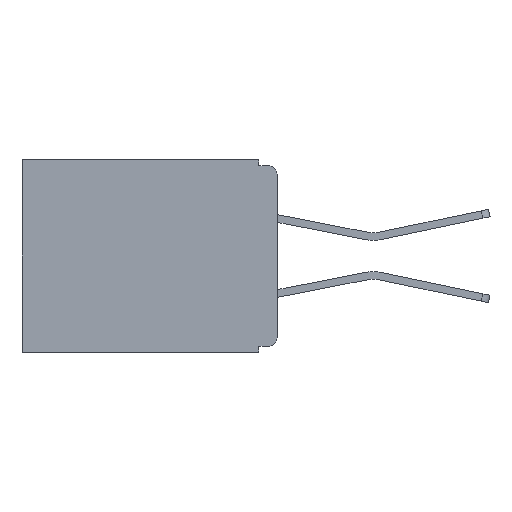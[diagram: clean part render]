
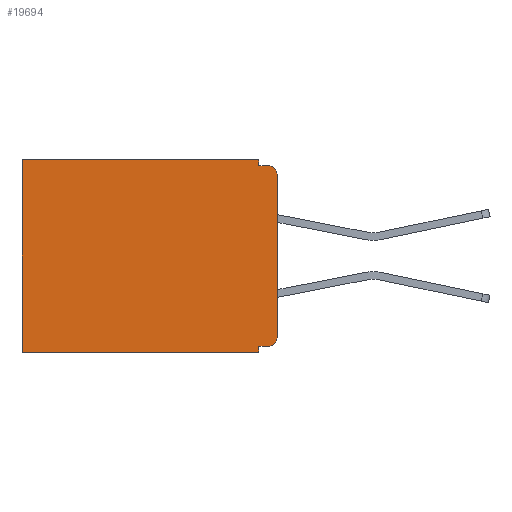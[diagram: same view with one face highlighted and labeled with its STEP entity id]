
A CAD part, left-side view. The second image highlights one B-rep face of the part: STEP entity #19694.
In plain terms, the highlighted planar face has unit normal (-1, 0, 0).
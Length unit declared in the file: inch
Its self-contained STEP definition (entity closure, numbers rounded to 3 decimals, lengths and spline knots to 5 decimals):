
#297 = CARTESIAN_POINT ( 'NONE',  ( 0.3, 0., -0.305 ) ) ;
#701 = LINE ( 'NONE', #4258, #16266 ) ;
#1469 = CARTESIAN_POINT ( 'NONE',  ( 0.3, 0.015, -0.025 ) ) ;
#2181 = DIRECTION ( 'NONE',  ( 0., -1., 0. ) ) ;
#2415 = VECTOR ( 'NONE', #14449, 39.37008 ) ;
#2641 = AXIS2_PLACEMENT_3D ( 'NONE', #9192, #23034, #11213 ) ;
#2864 = EDGE_CURVE ( 'NONE', #6134, #24382, #22647, .T. ) ;
#3348 = ORIENTED_EDGE ( 'NONE', *, *, #19267, .F. ) ;
#3487 = ORIENTED_EDGE ( 'NONE', *, *, #22700, .F. ) ;
#3613 = DIRECTION ( 'NONE',  ( 0., 0., -1. ) ) ;
#3929 = CARTESIAN_POINT ( 'NONE',  ( 0.3, 0., -0.33 ) ) ;
#4196 = ORIENTED_EDGE ( 'NONE', *, *, #20376, .T. ) ;
#4258 = CARTESIAN_POINT ( 'NONE',  ( 0.3, 0.031, -0.33 ) ) ;
#4679 = ORIENTED_EDGE ( 'NONE', *, *, #13429, .F. ) ;
#4730 = CARTESIAN_POINT ( 'NONE',  ( 0.3, 0.031, 0. ) ) ;
#5563 = ORIENTED_EDGE ( 'NONE', *, *, #15061, .T. ) ;
#5715 = LINE ( 'NONE', #25553, #11020 ) ;
#6134 = VERTEX_POINT ( 'NONE', #11916 ) ;
#6362 = DIRECTION ( 'NONE',  ( 0., 1., 0. ) ) ;
#6482 = CARTESIAN_POINT ( 'NONE',  ( 0.3, 0.437, -0.33 ) ) ;
#6527 = EDGE_LOOP ( 'NONE', ( #14852, #5563, #21403, #3348, #16487, #11966, #3487, #4679, #24324, #4196 ) ) ;
#6865 = VECTOR ( 'NONE', #13808, 39.37008 ) ;
#7107 = VECTOR ( 'NONE', #23859, 39.37008 ) ;
#7918 = LINE ( 'NONE', #6482, #2415 ) ;
#8064 = CARTESIAN_POINT ( 'NONE',  ( 0.3, 0.437, 0. ) ) ;
#8473 = VERTEX_POINT ( 'NONE', #13631 ) ;
#9192 = CARTESIAN_POINT ( 'NONE',  ( 0.3, 0., -0.33 ) ) ;
#9329 = CARTESIAN_POINT ( 'NONE',  ( 0.3, 0.015, -0.305 ) ) ;
#9375 = DIRECTION ( 'NONE',  ( 0., 1., 0. ) ) ;
#9679 = VECTOR ( 'NONE', #6362, 39.37008 ) ;
#9851 = AXIS2_PLACEMENT_3D ( 'NONE', #9329, #23171, #11361 ) ;
#11020 = VECTOR ( 'NONE', #15819, 39.37008 ) ;
#11213 = DIRECTION ( 'NONE',  ( 0., 0., -1. ) ) ;
#11361 = DIRECTION ( 'NONE',  ( 0., 0., -1. ) ) ;
#11678 = AXIS2_PLACEMENT_3D ( 'NONE', #1469, #15661, #3613 ) ;
#11916 = CARTESIAN_POINT ( 'NONE',  ( 0.3, 0.015, -0.32 ) ) ;
#11966 = ORIENTED_EDGE ( 'NONE', *, *, #18927, .T. ) ;
#12786 = VERTEX_POINT ( 'NONE', #8064 ) ;
#12873 = EDGE_CURVE ( 'NONE', #20831, #17509, #14748, .T. ) ;
#12981 = LINE ( 'NONE', #3929, #7107 ) ;
#13429 = EDGE_CURVE ( 'NONE', #24382, #20063, #701, .T. ) ;
#13631 = CARTESIAN_POINT ( 'NONE',  ( 0.3, 0.437, -0.33 ) ) ;
#13808 = DIRECTION ( 'NONE',  ( 0., 1., 0. ) ) ;
#13987 = CARTESIAN_POINT ( 'NONE',  ( 0.3, 0., -0.025 ) ) ;
#14298 = CARTESIAN_POINT ( 'NONE',  ( 0.3, 0., -0.32 ) ) ;
#14320 = CARTESIAN_POINT ( 'NONE',  ( 0.3, 0., -0.01 ) ) ;
#14449 = DIRECTION ( 'NONE',  ( 0., 0., -1. ) ) ;
#14748 = LINE ( 'NONE', #14320, #24571 ) ;
#14852 = ORIENTED_EDGE ( 'NONE', *, *, #17376, .F. ) ;
#14983 = LINE ( 'NONE', #20145, #9679 ) ;
#15061 = EDGE_CURVE ( 'NONE', #19309, #17509, #20521, .T. ) ;
#15650 = FACE_OUTER_BOUND ( 'NONE', #6527, .T. ) ;
#15661 = DIRECTION ( 'NONE',  ( -1., 0., 0. ) ) ;
#15819 = DIRECTION ( 'NONE',  ( 0., 0., -1. ) ) ;
#16266 = VECTOR ( 'NONE', #20239, 39.37008 ) ;
#16487 = ORIENTED_EDGE ( 'NONE', *, *, #21238, .T. ) ;
#16547 = CIRCLE ( 'NONE', #9851, 0.015 ) ;
#17376 = EDGE_CURVE ( 'NONE', #19309, #23676, #12981, .T. ) ;
#17509 = VERTEX_POINT ( 'NONE', #20367 ) ;
#18264 = VERTEX_POINT ( 'NONE', #4730 ) ;
#18927 = EDGE_CURVE ( 'NONE', #12786, #8473, #7918, .T. ) ;
#19142 = CARTESIAN_POINT ( 'NONE',  ( 0.3, 0.031, -0.32 ) ) ;
#19267 = EDGE_CURVE ( 'NONE', #18264, #20831, #5715, .T. ) ;
#19304 = CARTESIAN_POINT ( 'NONE',  ( 0.3, 0., -0.33 ) ) ;
#19309 = VERTEX_POINT ( 'NONE', #13987 ) ;
#19694 = ADVANCED_FACE ( 'NONE', ( #15650 ), #20994, .F. ) ;
#20063 = VERTEX_POINT ( 'NONE', #20378 ) ;
#20145 = CARTESIAN_POINT ( 'NONE',  ( 0.3, 0., 0. ) ) ;
#20239 = DIRECTION ( 'NONE',  ( 0., 0., -1. ) ) ;
#20367 = CARTESIAN_POINT ( 'NONE',  ( 0.3, 0.015, -0.01 ) ) ;
#20376 = EDGE_CURVE ( 'NONE', #6134, #23676, #16547, .T. ) ;
#20378 = CARTESIAN_POINT ( 'NONE',  ( 0.3, 0.031, -0.33 ) ) ;
#20521 = CIRCLE ( 'NONE', #11678, 0.015 ) ;
#20770 = CARTESIAN_POINT ( 'NONE',  ( 0.3, 0.031, -0.01 ) ) ;
#20831 = VERTEX_POINT ( 'NONE', #20770 ) ;
#20994 = PLANE ( 'NONE',  #2641 ) ;
#21238 = EDGE_CURVE ( 'NONE', #18264, #12786, #14983, .T. ) ;
#21403 = ORIENTED_EDGE ( 'NONE', *, *, #12873, .F. ) ;
#21699 = VECTOR ( 'NONE', #9375, 39.37008 ) ;
#22309 = LINE ( 'NONE', #19304, #21699 ) ;
#22647 = LINE ( 'NONE', #14298, #6865 ) ;
#22700 = EDGE_CURVE ( 'NONE', #20063, #8473, #22309, .T. ) ;
#23034 = DIRECTION ( 'NONE',  ( 1., 0., 0. ) ) ;
#23171 = DIRECTION ( 'NONE',  ( -1., 0., 0. ) ) ;
#23676 = VERTEX_POINT ( 'NONE', #297 ) ;
#23859 = DIRECTION ( 'NONE',  ( 0., 0., -1. ) ) ;
#24324 = ORIENTED_EDGE ( 'NONE', *, *, #2864, .F. ) ;
#24382 = VERTEX_POINT ( 'NONE', #19142 ) ;
#24571 = VECTOR ( 'NONE', #2181, 39.37008 ) ;
#25553 = CARTESIAN_POINT ( 'NONE',  ( 0.3, 0.031, 0. ) ) ;
